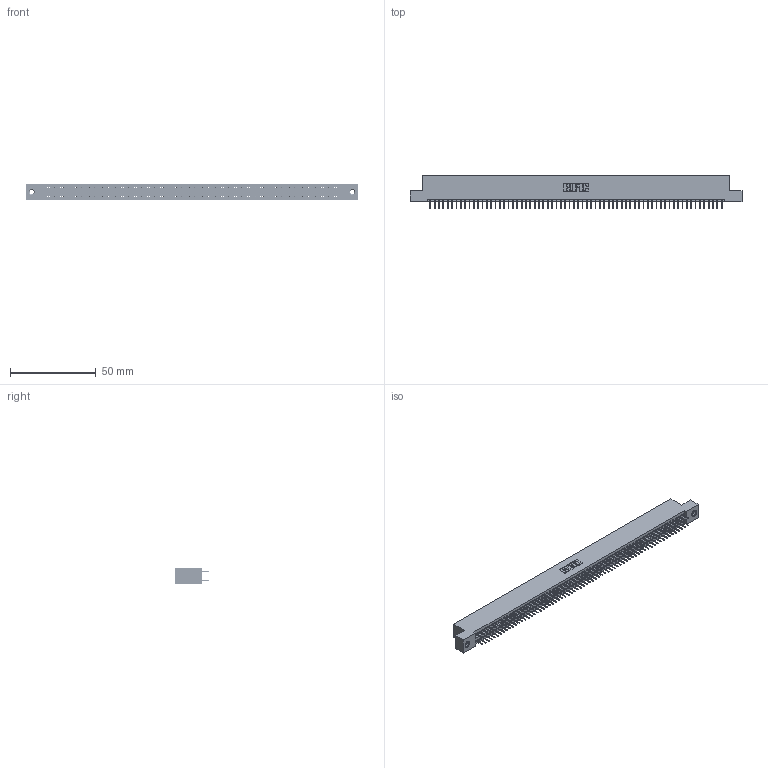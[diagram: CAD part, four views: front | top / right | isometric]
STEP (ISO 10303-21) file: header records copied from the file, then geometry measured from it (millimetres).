
FILE_DESCRIPTION (( 'STEP AP203' ), '1' );
FILE_NAME ('345-136-524-207.STEP', '2019-11-08T07:36:36', ( '' ), ( '' ), 'SwSTEP 2.0', 'SolidWorks 2016', '' );
FILE_SCHEMA (( 'CONFIG_CONTROL_DESIGN' ));
Length unit declared in the file: inch
Products named in the file (4): 345-292-001_345-293-124; 345 Part_Flush Mounting Lugs - 0.156 Dia-TI; 345-136-524-207; 345-250-001_345-250-005-103
Assembly tree (139 placements, depth 2):
  345-136-524-207
    345 Part_Flush Mounting Lugs - 0.156 Dia-TI
    345-292-001_345-293-124  x136
    345-250-001_345-250-005-103  x2
Bounding box: 193.93 x 19.35 x 9.4 mm (x, y, z)
Volume: 18860.5 mm3; surface area: 27867.1 mm2
Topology: 139 solids, 139 shells, 7530 faces, 21285 edges, 13638 vertices
Faces by surface type: plane 5416, cylinder 2098, cone 12, torus 4
Entity records: 51114 total; most frequent: CARTESIAN_POINT 8523, ORIENTED_EDGE 8450, DIRECTION 7511, EDGE_CURVE 4225, LINE 3805, VECTOR 3805, VERTEX_POINT 2808, AXIS2_PLACEMENT_3D 1853
